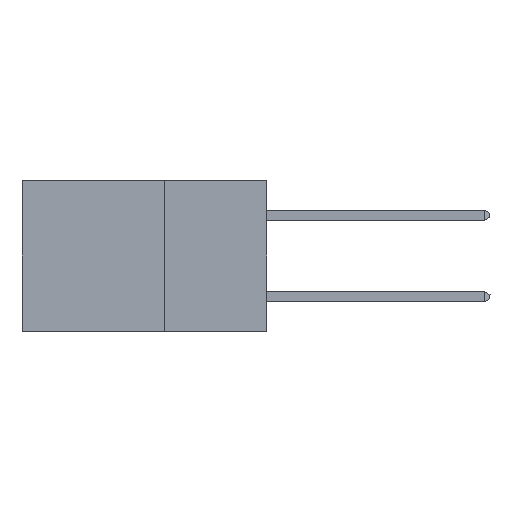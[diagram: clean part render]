
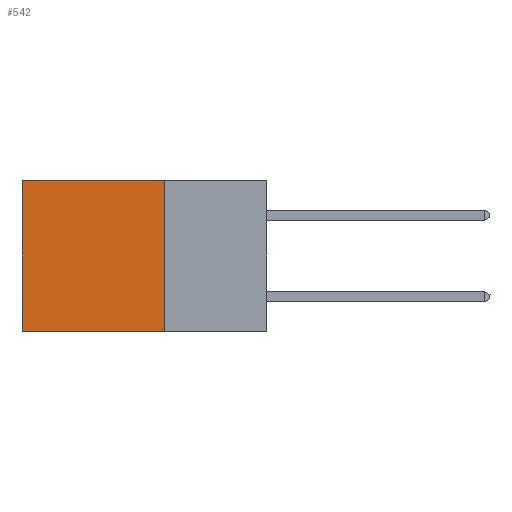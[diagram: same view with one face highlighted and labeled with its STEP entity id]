
A CAD part, left-side view. The second image highlights one B-rep face of the part: STEP entity #542.
In plain terms, the highlighted planar face has unit normal (-1, 0, 0).
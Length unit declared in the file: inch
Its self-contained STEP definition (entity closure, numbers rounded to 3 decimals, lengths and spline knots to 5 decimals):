
#446 = DIRECTION ( 'NONE',  ( 0., 0., -1. ) ) ;
#542 = ADVANCED_FACE ( 'NONE', ( #6450 ), #7287, .F. ) ;
#547 = VERTEX_POINT ( 'NONE', #3078 ) ;
#993 = ORIENTED_EDGE ( 'NONE', *, *, #2556, .F. ) ;
#1947 = VERTEX_POINT ( 'NONE', #6287 ) ;
#2556 = EDGE_CURVE ( 'NONE', #1947, #3781, #7592, .T. ) ;
#2694 = EDGE_CURVE ( 'NONE', #3781, #547, #12131, .T. ) ;
#2701 = CARTESIAN_POINT ( 'NONE',  ( 0.2875, 0.6, 0. ) ) ;
#3078 = CARTESIAN_POINT ( 'NONE',  ( 0.2875, 0.6, -0.37 ) ) ;
#3152 = CARTESIAN_POINT ( 'NONE',  ( 0.2875, 0.25, 0. ) ) ;
#3781 = VERTEX_POINT ( 'NONE', #7809 ) ;
#4190 = DIRECTION ( 'NONE',  ( 0., 1., 0. ) ) ;
#4258 = DIRECTION ( 'NONE',  ( 1., 0., 0. ) ) ;
#4347 = CARTESIAN_POINT ( 'NONE',  ( 0.2875, 0.6, 0. ) ) ;
#5564 = ORIENTED_EDGE ( 'NONE', *, *, #7317, .T. ) ;
#6007 = ORIENTED_EDGE ( 'NONE', *, *, #12450, .T. ) ;
#6287 = CARTESIAN_POINT ( 'NONE',  ( 0.2875, 0.25, 0. ) ) ;
#6450 = FACE_OUTER_BOUND ( 'NONE', #13022, .T. ) ;
#7003 = DIRECTION ( 'NONE',  ( 0., 1., 0. ) ) ;
#7161 = LINE ( 'NONE', #7232, #9501 ) ;
#7232 = CARTESIAN_POINT ( 'NONE',  ( 0.2875, 0.25, 0. ) ) ;
#7278 = VECTOR ( 'NONE', #8765, 39.37008 ) ;
#7287 = PLANE ( 'NONE',  #13237 ) ;
#7317 = EDGE_CURVE ( 'NONE', #1947, #11747, #7161, .T. ) ;
#7592 = LINE ( 'NONE', #10979, #7278 ) ;
#7809 = CARTESIAN_POINT ( 'NONE',  ( 0.2875, 0.25, -0.37 ) ) ;
#8765 = DIRECTION ( 'NONE',  ( 0., 0., -1. ) ) ;
#9501 = VECTOR ( 'NONE', #7003, 39.37008 ) ;
#10023 = VECTOR ( 'NONE', #12765, 39.37008 ) ;
#10346 = VECTOR ( 'NONE', #4190, 39.37008 ) ;
#10489 = LINE ( 'NONE', #2701, #10023 ) ;
#10979 = CARTESIAN_POINT ( 'NONE',  ( 0.2875, 0.25, 0. ) ) ;
#11074 = ORIENTED_EDGE ( 'NONE', *, *, #2694, .F. ) ;
#11747 = VERTEX_POINT ( 'NONE', #4347 ) ;
#12131 = LINE ( 'NONE', #13303, #10346 ) ;
#12450 = EDGE_CURVE ( 'NONE', #11747, #547, #10489, .T. ) ;
#12765 = DIRECTION ( 'NONE',  ( 0., 0., -1. ) ) ;
#13022 = EDGE_LOOP ( 'NONE', ( #6007, #11074, #993, #5564 ) ) ;
#13237 = AXIS2_PLACEMENT_3D ( 'NONE', #3152, #4258, #446 ) ;
#13303 = CARTESIAN_POINT ( 'NONE',  ( 0.2875, 0.25, -0.37 ) ) ;
